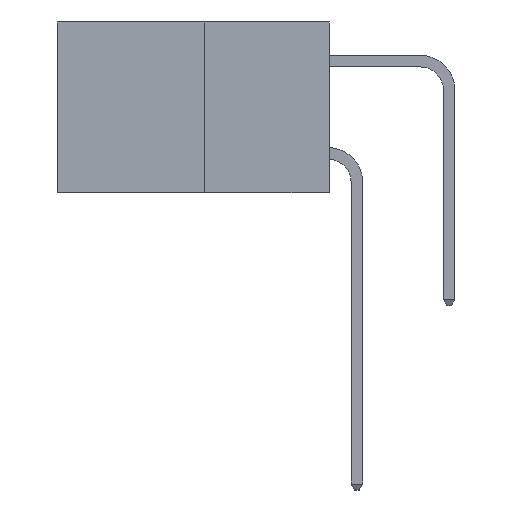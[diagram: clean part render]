
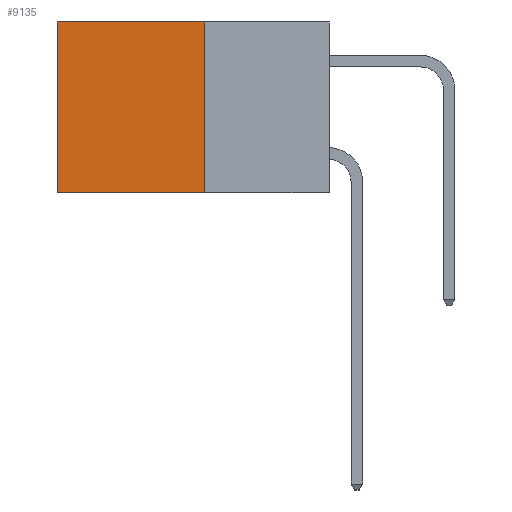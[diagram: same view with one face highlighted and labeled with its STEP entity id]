
A CAD part, left-side view. The second image highlights one B-rep face of the part: STEP entity #9135.
In plain terms, the highlighted planar face has unit normal (-1, 0, 0).
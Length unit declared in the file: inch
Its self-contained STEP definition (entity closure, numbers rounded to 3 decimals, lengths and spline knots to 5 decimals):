
#600 = CARTESIAN_POINT ( 'NONE',  ( 0.277, 0.27, -0.37 ) ) ;
#874 = CARTESIAN_POINT ( 'NONE',  ( 0.277, 0.59, 0. ) ) ;
#1951 = EDGE_CURVE ( 'NONE', #13907, #8462, #4399, .T. ) ;
#2180 = LINE ( 'NONE', #7466, #11363 ) ;
#2419 = VECTOR ( 'NONE', #10311, 39.37008 ) ;
#2586 = LINE ( 'NONE', #4191, #11742 ) ;
#2806 = LINE ( 'NONE', #7877, #2419 ) ;
#3821 = DIRECTION ( 'NONE',  ( 0., 0., -1. ) ) ;
#4029 = VECTOR ( 'NONE', #4043, 39.37008 ) ;
#4043 = DIRECTION ( 'NONE',  ( 0., 1., 0. ) ) ;
#4191 = CARTESIAN_POINT ( 'NONE',  ( 0.277, 0.27, -0.37 ) ) ;
#4399 = LINE ( 'NONE', #9878, #4029 ) ;
#4766 = ORIENTED_EDGE ( 'NONE', *, *, #12668, .F. ) ;
#6092 = VERTEX_POINT ( 'NONE', #874 ) ;
#7034 = CARTESIAN_POINT ( 'NONE',  ( 0.277, 0.27, 0. ) ) ;
#7466 = CARTESIAN_POINT ( 'NONE',  ( 0.277, 0.27, 0. ) ) ;
#7734 = VERTEX_POINT ( 'NONE', #7034 ) ;
#7877 = CARTESIAN_POINT ( 'NONE',  ( 0.277, 0.59, -0.37 ) ) ;
#8462 = VERTEX_POINT ( 'NONE', #14321 ) ;
#8528 = AXIS2_PLACEMENT_3D ( 'NONE', #9822, #11000, #3821 ) ;
#8608 = PLANE ( 'NONE',  #8528 ) ;
#8649 = DIRECTION ( 'NONE',  ( 0., 1., 0. ) ) ;
#9135 = ADVANCED_FACE ( 'NONE', ( #14565 ), #8608, .F. ) ;
#9255 = EDGE_LOOP ( 'NONE', ( #13559, #12322, #4766, #15204 ) ) ;
#9822 = CARTESIAN_POINT ( 'NONE',  ( 0.277, 0.27, -0.37 ) ) ;
#9878 = CARTESIAN_POINT ( 'NONE',  ( 0.277, 0.27, -0.37 ) ) ;
#10311 = DIRECTION ( 'NONE',  ( 0., 0., -1. ) ) ;
#11000 = DIRECTION ( 'NONE',  ( 1., 0., 0. ) ) ;
#11363 = VECTOR ( 'NONE', #8649, 39.37008 ) ;
#11742 = VECTOR ( 'NONE', #13716, 39.37008 ) ;
#12322 = ORIENTED_EDGE ( 'NONE', *, *, #1951, .F. ) ;
#12668 = EDGE_CURVE ( 'NONE', #7734, #13907, #2586, .T. ) ;
#13137 = EDGE_CURVE ( 'NONE', #7734, #6092, #2180, .T. ) ;
#13559 = ORIENTED_EDGE ( 'NONE', *, *, #13955, .T. ) ;
#13716 = DIRECTION ( 'NONE',  ( 0., 0., -1. ) ) ;
#13907 = VERTEX_POINT ( 'NONE', #600 ) ;
#13955 = EDGE_CURVE ( 'NONE', #6092, #8462, #2806, .T. ) ;
#14321 = CARTESIAN_POINT ( 'NONE',  ( 0.277, 0.59, -0.37 ) ) ;
#14565 = FACE_OUTER_BOUND ( 'NONE', #9255, .T. ) ;
#15204 = ORIENTED_EDGE ( 'NONE', *, *, #13137, .T. ) ;
